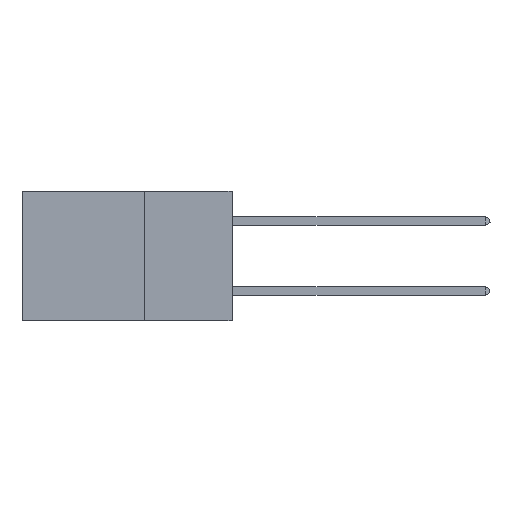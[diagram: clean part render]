
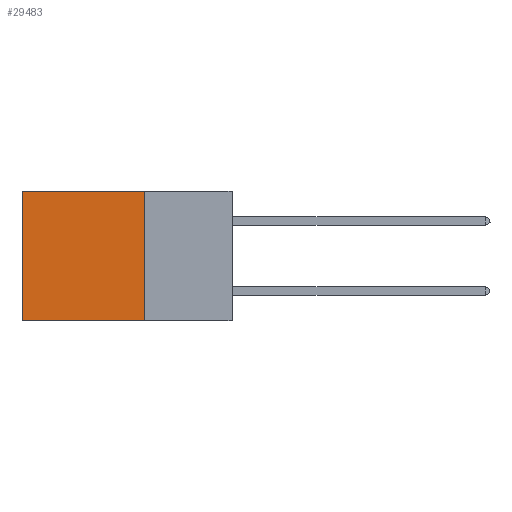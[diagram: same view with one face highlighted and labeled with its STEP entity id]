
A CAD part, left-side view. The second image highlights one B-rep face of the part: STEP entity #29483.
In plain terms, the highlighted planar face has unit normal (-1, 0, 0).
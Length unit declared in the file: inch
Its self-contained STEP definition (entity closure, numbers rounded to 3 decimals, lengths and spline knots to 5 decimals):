
#4 = ORIENTED_EDGE ( 'NONE', *, *, #30914, .T. ) ;
#283 = DIRECTION ( 'NONE',  ( 0., 1., 0. ) ) ;
#1944 = DIRECTION ( 'NONE',  ( 0., 0., -1. ) ) ;
#3832 = VECTOR ( 'NONE', #33261, 39.37008 ) ;
#5364 = VERTEX_POINT ( 'NONE', #24662 ) ;
#5608 = LINE ( 'NONE', #6033, #20121 ) ;
#6022 = CARTESIAN_POINT ( 'NONE',  ( 0.2875, 0.25, -0.37 ) ) ;
#6033 = CARTESIAN_POINT ( 'NONE',  ( 0.2875, 0.6, 0. ) ) ;
#6345 = LINE ( 'NONE', #20184, #3832 ) ;
#6796 = ORIENTED_EDGE ( 'NONE', *, *, #30303, .T. ) ;
#7036 = LINE ( 'NONE', #21379, #16606 ) ;
#8148 = CARTESIAN_POINT ( 'NONE',  ( 0.2875, 0.6, 0. ) ) ;
#9989 = ORIENTED_EDGE ( 'NONE', *, *, #16077, .F. ) ;
#14587 = LINE ( 'NONE', #20733, #24171 ) ;
#15392 = CARTESIAN_POINT ( 'NONE',  ( 0.2875, 0.25, 0. ) ) ;
#15869 = VERTEX_POINT ( 'NONE', #8148 ) ;
#16077 = EDGE_CURVE ( 'NONE', #19932, #29993, #6345, .T. ) ;
#16606 = VECTOR ( 'NONE', #283, 39.37008 ) ;
#16764 = AXIS2_PLACEMENT_3D ( 'NONE', #15392, #26504, #31370 ) ;
#18555 = CARTESIAN_POINT ( 'NONE',  ( 0.2875, 0.6, -0.37 ) ) ;
#19932 = VERTEX_POINT ( 'NONE', #6022 ) ;
#20121 = VECTOR ( 'NONE', #32566, 39.37008 ) ;
#20184 = CARTESIAN_POINT ( 'NONE',  ( 0.2875, 0.25, -0.37 ) ) ;
#20733 = CARTESIAN_POINT ( 'NONE',  ( 0.2875, 0.25, 0. ) ) ;
#21014 = FACE_OUTER_BOUND ( 'NONE', #22009, .T. ) ;
#21379 = CARTESIAN_POINT ( 'NONE',  ( 0.2875, 0.25, 0. ) ) ;
#22009 = EDGE_LOOP ( 'NONE', ( #6796, #9989, #28345, #4 ) ) ;
#22274 = EDGE_CURVE ( 'NONE', #5364, #19932, #14587, .T. ) ;
#24171 = VECTOR ( 'NONE', #1944, 39.37008 ) ;
#24662 = CARTESIAN_POINT ( 'NONE',  ( 0.2875, 0.25, 0. ) ) ;
#26504 = DIRECTION ( 'NONE',  ( 1., 0., 0. ) ) ;
#28345 = ORIENTED_EDGE ( 'NONE', *, *, #22274, .F. ) ;
#28815 = PLANE ( 'NONE',  #16764 ) ;
#29483 = ADVANCED_FACE ( 'NONE', ( #21014 ), #28815, .F. ) ;
#29993 = VERTEX_POINT ( 'NONE', #18555 ) ;
#30303 = EDGE_CURVE ( 'NONE', #15869, #29993, #5608, .T. ) ;
#30914 = EDGE_CURVE ( 'NONE', #5364, #15869, #7036, .T. ) ;
#31370 = DIRECTION ( 'NONE',  ( 0., 0., -1. ) ) ;
#32566 = DIRECTION ( 'NONE',  ( 0., 0., -1. ) ) ;
#33261 = DIRECTION ( 'NONE',  ( 0., 1., 0. ) ) ;
